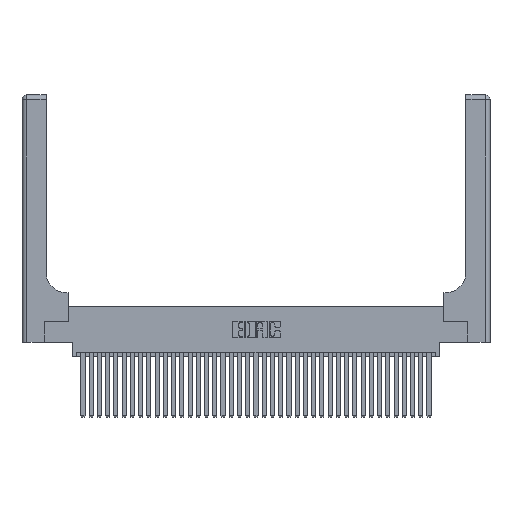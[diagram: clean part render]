
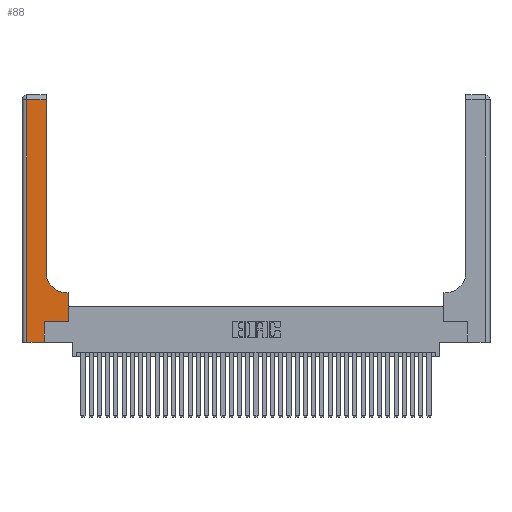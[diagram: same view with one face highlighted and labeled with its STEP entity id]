
A CAD part, top view. The second image highlights one B-rep face of the part: STEP entity #88.
In plain terms, the highlighted planar face has unit normal (0, 0, 1).
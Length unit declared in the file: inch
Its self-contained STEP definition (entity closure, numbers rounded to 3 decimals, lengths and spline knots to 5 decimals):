
#88 = ADVANCED_FACE ( 'NONE', ( #9979 ), #19882, .F. ) ;
#2294 = EDGE_CURVE ( 'NONE', #28897, #11949, #9830, .T. ) ;
#3942 = DIRECTION ( 'NONE',  ( 0., 1., 0. ) ) ;
#4012 = VECTOR ( 'NONE', #20120, 39.37008 ) ;
#4123 = CARTESIAN_POINT ( 'NONE',  ( 0.2915, 0.6, 0.37 ) ) ;
#4762 = ORIENTED_EDGE ( 'NONE', *, *, #37664, .T. ) ;
#4789 = CARTESIAN_POINT ( 'NONE',  ( 0.2915, 2.94, 0.37 ) ) ;
#6424 = CARTESIAN_POINT ( 'NONE',  ( 0.5585, 0.25, 0.37 ) ) ;
#6549 = EDGE_CURVE ( 'NONE', #37160, #24481, #14301, .T. ) ;
#7071 = VERTEX_POINT ( 'NONE', #4789 ) ;
#7357 = DIRECTION ( 'NONE',  ( 1., 0., 0. ) ) ;
#7499 = DIRECTION ( 'NONE',  ( -1., 0., 0. ) ) ;
#7605 = CARTESIAN_POINT ( 'NONE',  ( 0., 0., 0.37 ) ) ;
#8800 = VECTOR ( 'NONE', #18784, 39.37008 ) ;
#9315 = CARTESIAN_POINT ( 'NONE',  ( 0.06, 0., 0.37 ) ) ;
#9830 = LINE ( 'NONE', #11233, #32744 ) ;
#9979 = FACE_OUTER_BOUND ( 'NONE', #10166, .T. ) ;
#10161 = VERTEX_POINT ( 'NONE', #33844 ) ;
#10166 = EDGE_LOOP ( 'NONE', ( #23400, #30375, #36509, #4762, #16691, #20308, #35906, #34610, #12128 ) ) ;
#10820 = CARTESIAN_POINT ( 'NONE',  ( 0., 2.94, 0.37 ) ) ;
#10838 = VERTEX_POINT ( 'NONE', #21837 ) ;
#11178 = CARTESIAN_POINT ( 'NONE',  ( 0.2915, 3., 0.37 ) ) ;
#11233 = CARTESIAN_POINT ( 'NONE',  ( 0.269, 0.25, 0.37 ) ) ;
#11949 = VERTEX_POINT ( 'NONE', #31982 ) ;
#12128 = ORIENTED_EDGE ( 'NONE', *, *, #17777, .T. ) ;
#13173 = VECTOR ( 'NONE', #27161, 39.37008 ) ;
#14082 = DIRECTION ( 'NONE',  ( 1., 0., 0. ) ) ;
#14301 = LINE ( 'NONE', #30603, #8800 ) ;
#14715 = DIRECTION ( 'NONE',  ( -1., 0., 0. ) ) ;
#15040 = CIRCLE ( 'NONE', #25628, 0.25 ) ;
#16691 = ORIENTED_EDGE ( 'NONE', *, *, #27384, .T. ) ;
#16705 = CARTESIAN_POINT ( 'NONE',  ( 0.06, 2.94, 0.37 ) ) ;
#17039 = EDGE_CURVE ( 'NONE', #11949, #10838, #33357, .T. ) ;
#17777 = EDGE_CURVE ( 'NONE', #27133, #27343, #15040, .T. ) ;
#17939 = LINE ( 'NONE', #10820, #4012 ) ;
#18091 = VECTOR ( 'NONE', #7357, 39.37008 ) ;
#18784 = DIRECTION ( 'NONE',  ( 0., -1., 0. ) ) ;
#19882 = PLANE ( 'NONE',  #21383 ) ;
#20120 = DIRECTION ( 'NONE',  ( -1., 0., 0. ) ) ;
#20308 = ORIENTED_EDGE ( 'NONE', *, *, #2294, .T. ) ;
#21383 = AXIS2_PLACEMENT_3D ( 'NONE', #22897, #29086, #14715 ) ;
#21420 = LINE ( 'NONE', #4123, #32763 ) ;
#21648 = LINE ( 'NONE', #11178, #24941 ) ;
#21837 = CARTESIAN_POINT ( 'NONE',  ( 0.5585, 0.6, 0.37 ) ) ;
#22278 = EDGE_CURVE ( 'NONE', #7071, #37160, #17939, .T. ) ;
#22897 = CARTESIAN_POINT ( 'NONE',  ( 0., 3., 0.37 ) ) ;
#23400 = ORIENTED_EDGE ( 'NONE', *, *, #25459, .T. ) ;
#24243 = CARTESIAN_POINT ( 'NONE',  ( 0.269, 0., 0.37 ) ) ;
#24481 = VERTEX_POINT ( 'NONE', #9315 ) ;
#24941 = VECTOR ( 'NONE', #25925, 39.37008 ) ;
#25045 = CARTESIAN_POINT ( 'NONE',  ( 0.5415, 0.6, 0.37 ) ) ;
#25243 = DIRECTION ( 'NONE',  ( 0., 0., -1. ) ) ;
#25459 = EDGE_CURVE ( 'NONE', #27343, #7071, #21648, .T. ) ;
#25628 = AXIS2_PLACEMENT_3D ( 'NONE', #38303, #25243, #37721 ) ;
#25925 = DIRECTION ( 'NONE',  ( 0., 1., 0. ) ) ;
#26062 = LINE ( 'NONE', #7605, #18091 ) ;
#27133 = VERTEX_POINT ( 'NONE', #25045 ) ;
#27161 = DIRECTION ( 'NONE',  ( 0., 1., 0. ) ) ;
#27343 = VERTEX_POINT ( 'NONE', #37667 ) ;
#27384 = EDGE_CURVE ( 'NONE', #10161, #28897, #30024, .T. ) ;
#28897 = VERTEX_POINT ( 'NONE', #34270 ) ;
#28903 = EDGE_CURVE ( 'NONE', #10838, #27133, #21420, .T. ) ;
#29086 = DIRECTION ( 'NONE',  ( 0., 0., -1. ) ) ;
#30024 = LINE ( 'NONE', #24243, #13173 ) ;
#30375 = ORIENTED_EDGE ( 'NONE', *, *, #22278, .T. ) ;
#30603 = CARTESIAN_POINT ( 'NONE',  ( 0.06, 3., 0.37 ) ) ;
#31982 = CARTESIAN_POINT ( 'NONE',  ( 0.5585, 0.25, 0.37 ) ) ;
#32744 = VECTOR ( 'NONE', #14082, 39.37008 ) ;
#32763 = VECTOR ( 'NONE', #7499, 39.37008 ) ;
#32896 = VECTOR ( 'NONE', #3942, 39.37008 ) ;
#33357 = LINE ( 'NONE', #6424, #32896 ) ;
#33844 = CARTESIAN_POINT ( 'NONE',  ( 0.269, 0., 0.37 ) ) ;
#34270 = CARTESIAN_POINT ( 'NONE',  ( 0.269, 0.25, 0.37 ) ) ;
#34610 = ORIENTED_EDGE ( 'NONE', *, *, #28903, .T. ) ;
#35906 = ORIENTED_EDGE ( 'NONE', *, *, #17039, .T. ) ;
#36509 = ORIENTED_EDGE ( 'NONE', *, *, #6549, .T. ) ;
#37160 = VERTEX_POINT ( 'NONE', #16705 ) ;
#37664 = EDGE_CURVE ( 'NONE', #24481, #10161, #26062, .T. ) ;
#37667 = CARTESIAN_POINT ( 'NONE',  ( 0.2915, 0.85, 0.37 ) ) ;
#37721 = DIRECTION ( 'NONE',  ( 1., 0., 0. ) ) ;
#38303 = CARTESIAN_POINT ( 'NONE',  ( 0.5415, 0.85, 0.37 ) ) ;
